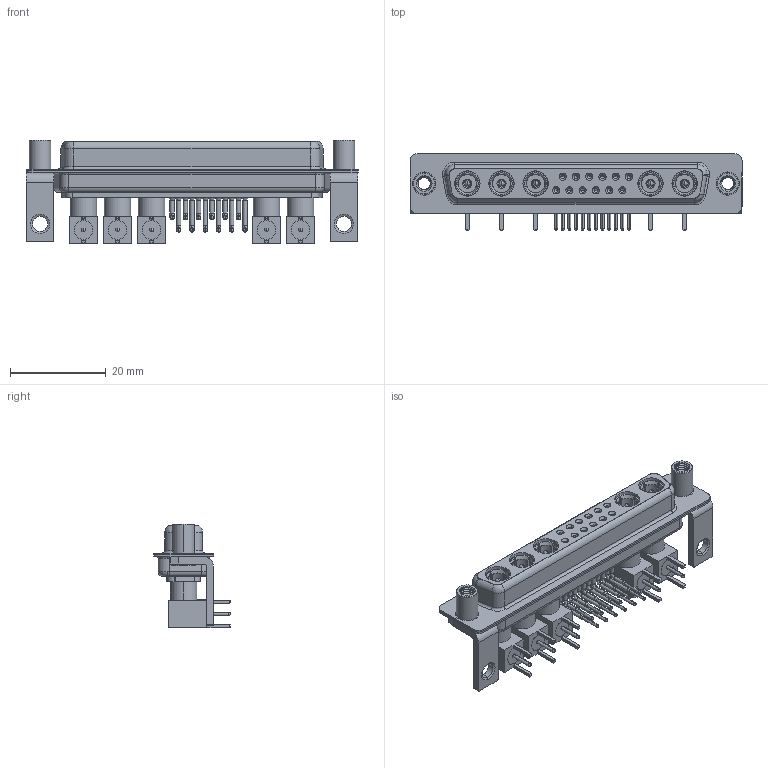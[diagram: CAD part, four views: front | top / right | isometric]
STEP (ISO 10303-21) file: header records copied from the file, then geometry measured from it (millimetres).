
FILE_DESCRIPTION (( 'STEP AP203' ), '1' );
FILE_NAME ('630-17W5640-5TE.STEP', '2022-06-06T23:39:04', ( '' ), ( '' ), 'SwSTEP 2.0', 'SolidWorks 2020', '' );
FILE_SCHEMA (( 'CONFIG_CONTROL_DESIGN' ));
Length unit declared in the file: millimetre
Products named in the file (19): Locking Collar; Pin_RA; Co-Ax Plug Assy_RA; 630Combo Threaded Standoff_D; Co-Ax Plug_RA PC Tail; 630-17W5640-5TE; 630Combo Housing_17W5; 630Combo Shell Front_37 Contacts; Insulator RA Pin; 630Combo Contact Row 1; 630Combo Contact Row 2; 630Combo Stabilizer Bracket; Insulator Pin_Straight PC Tail; RA Back Shell; 630Combo Shell Rear_37 Contacts
Assembly tree (54 placements, depth 3):
  630-17W5640-5TE
    630Combo Housing_17W5
    630Combo Shell Front_37 Contacts
    630Combo Shell Rear_37 Contacts
    630Combo Stabilizer Bracket  x2
    630Combo Threaded Standoff_D  x2
    Co-Ax Plug Assy_RA
      Co-Ax Plug_RA PC Tail
      Insulator Pin_Straight PC Tail
      Pin_RA
      Locking Collar
      RA Back Shell
      Insulator RA Pin
    Co-Ax Plug Assy_RA
      Co-Ax Plug_RA PC Tail
      Insulator Pin_Straight PC Tail
      Pin_RA
      Locking Collar
      RA Back Shell
      Insulator RA Pin
    Co-Ax Plug Assy_RA
      Co-Ax Plug_RA PC Tail
      Insulator Pin_Straight PC Tail
      Pin_RA
      Locking Collar
      RA Back Shell
      Insulator RA Pin
    Co-Ax Plug Assy_RA
      Co-Ax Plug_RA PC Tail
      Insulator Pin_Straight PC Tail
      Pin_RA
      Locking Collar
      RA Back Shell
      Insulator RA Pin
    Co-Ax Plug Assy_RA
      Co-Ax Plug_RA PC Tail
      Insulator Pin_Straight PC Tail
      Pin_RA
      Locking Collar
      RA Back Shell
      Insulator RA Pin
    630Combo Contact Row 1  x6
    630Combo Contact Row 2  x6
Bounding box: 69.4 x 16 x 21.61 mm (x, y, z)
Volume: 6887 mm3; surface area: 16416.1 mm2
Topology: 49 solids, 49 shells, 1853 faces, 4580 edges, 2880 vertices
Faces by surface type: cylinder 810, plane 604, cone 273, torus 87, bspline 59, sphere 20
Entity records: 26832 total; most frequent: CARTESIAN_POINT 6519, DIRECTION 3934, ORIENTED_EDGE 3436, EDGE_CURVE 1718, AXIS2_PLACEMENT_3D 1609, VERTEX_POINT 1095, EDGE_LOOP 849, CIRCLE 840
